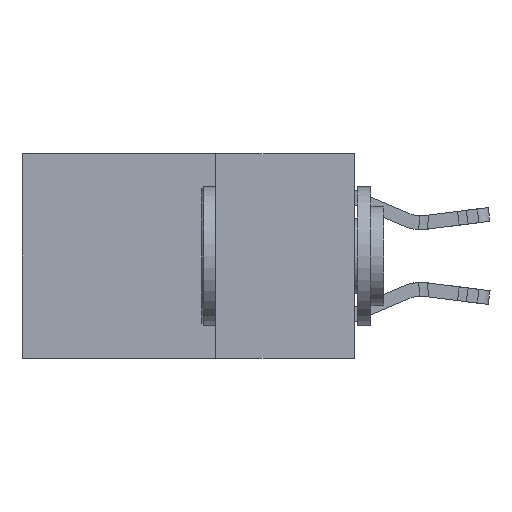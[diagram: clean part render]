
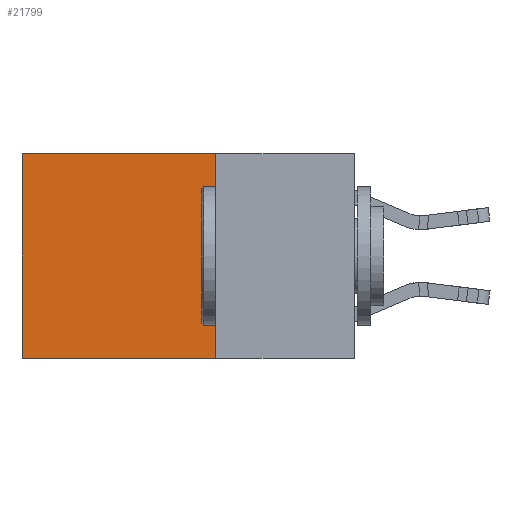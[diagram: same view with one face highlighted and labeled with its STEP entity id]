
A CAD part, left-side view. The second image highlights one B-rep face of the part: STEP entity #21799.
In plain terms, the highlighted planar face has unit normal (-1, 0, 0).
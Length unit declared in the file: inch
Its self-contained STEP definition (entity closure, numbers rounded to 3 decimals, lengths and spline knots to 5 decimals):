
#866 = LINE ( 'NONE', #2247, #24458 ) ;
#1900 = CARTESIAN_POINT ( 'NONE',  ( 0.2625, 0.6, 0. ) ) ;
#2247 = CARTESIAN_POINT ( 'NONE',  ( 0.2625, 0.25, -0.37 ) ) ;
#2965 = DIRECTION ( 'NONE',  ( 0., 0., -1. ) ) ;
#4326 = ORIENTED_EDGE ( 'NONE', *, *, #17575, .T. ) ;
#5789 = ORIENTED_EDGE ( 'NONE', *, *, #16586, .F. ) ;
#7084 = VERTEX_POINT ( 'NONE', #11242 ) ;
#7975 = AXIS2_PLACEMENT_3D ( 'NONE', #22459, #24828, #11243 ) ;
#9455 = LINE ( 'NONE', #1900, #26133 ) ;
#9702 = VECTOR ( 'NONE', #22137, 39.37008 ) ;
#11125 = DIRECTION ( 'NONE',  ( 0., 0., -1. ) ) ;
#11242 = CARTESIAN_POINT ( 'NONE',  ( 0.2625, 0.25, 0. ) ) ;
#11243 = DIRECTION ( 'NONE',  ( 0., 0., -1. ) ) ;
#11862 = ORIENTED_EDGE ( 'NONE', *, *, #27211, .F. ) ;
#12620 = FACE_OUTER_BOUND ( 'NONE', #29104, .T. ) ;
#12912 = EDGE_CURVE ( 'NONE', #7084, #16075, #27766, .T. ) ;
#13571 = VERTEX_POINT ( 'NONE', #19787 ) ;
#14399 = CARTESIAN_POINT ( 'NONE',  ( 0.2625, 0.25, 0. ) ) ;
#15354 = CARTESIAN_POINT ( 'NONE',  ( 0.2625, 0.25, 0. ) ) ;
#16075 = VERTEX_POINT ( 'NONE', #27509 ) ;
#16586 = EDGE_CURVE ( 'NONE', #25174, #13571, #866, .T. ) ;
#17575 = EDGE_CURVE ( 'NONE', #16075, #13571, #9455, .T. ) ;
#19787 = CARTESIAN_POINT ( 'NONE',  ( 0.2625, 0.6, -0.37 ) ) ;
#20697 = VECTOR ( 'NONE', #2965, 39.37008 ) ;
#21799 = ADVANCED_FACE ( 'NONE', ( #12620 ), #29193, .F. ) ;
#22137 = DIRECTION ( 'NONE',  ( 0., 1., 0. ) ) ;
#22459 = CARTESIAN_POINT ( 'NONE',  ( 0.2625, 0.25, 0. ) ) ;
#22777 = DIRECTION ( 'NONE',  ( 0., 1., 0. ) ) ;
#24458 = VECTOR ( 'NONE', #22777, 39.37008 ) ;
#24641 = ORIENTED_EDGE ( 'NONE', *, *, #12912, .T. ) ;
#24828 = DIRECTION ( 'NONE',  ( 1., 0., 0. ) ) ;
#25174 = VERTEX_POINT ( 'NONE', #27556 ) ;
#26133 = VECTOR ( 'NONE', #11125, 39.37008 ) ;
#26675 = LINE ( 'NONE', #14399, #20697 ) ;
#27211 = EDGE_CURVE ( 'NONE', #7084, #25174, #26675, .T. ) ;
#27509 = CARTESIAN_POINT ( 'NONE',  ( 0.2625, 0.6, 0. ) ) ;
#27556 = CARTESIAN_POINT ( 'NONE',  ( 0.2625, 0.25, -0.37 ) ) ;
#27766 = LINE ( 'NONE', #15354, #9702 ) ;
#29104 = EDGE_LOOP ( 'NONE', ( #4326, #5789, #11862, #24641 ) ) ;
#29193 = PLANE ( 'NONE',  #7975 ) ;
